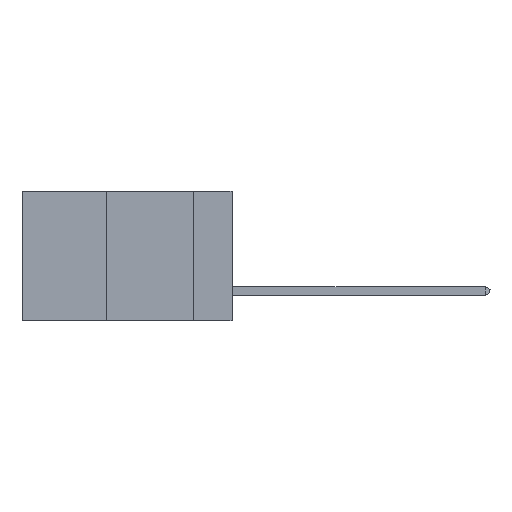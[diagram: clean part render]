
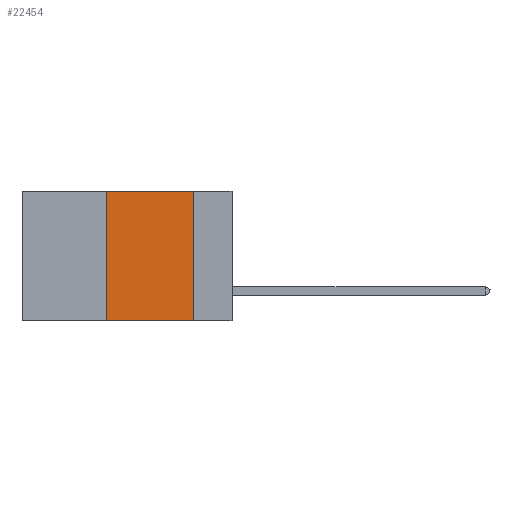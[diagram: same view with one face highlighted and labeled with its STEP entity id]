
A CAD part, left-side view. The second image highlights one B-rep face of the part: STEP entity #22454.
In plain terms, the highlighted planar face has unit normal (-1, 0, 0).
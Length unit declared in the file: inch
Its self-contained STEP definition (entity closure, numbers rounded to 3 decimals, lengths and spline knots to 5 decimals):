
#718 = AXIS2_PLACEMENT_3D ( 'NONE', #11812, #4247, #4159 ) ;
#1713 = VECTOR ( 'NONE', #14439, 39.37008 ) ;
#2725 = VERTEX_POINT ( 'NONE', #11721 ) ;
#4064 = DIRECTION ( 'NONE',  ( 0., 0., -1. ) ) ;
#4159 = DIRECTION ( 'NONE',  ( 0., 0., -1. ) ) ;
#4247 = DIRECTION ( 'NONE',  ( 1., 0., 0. ) ) ;
#4410 = PLANE ( 'NONE',  #718 ) ;
#4430 = VERTEX_POINT ( 'NONE', #20832 ) ;
#6059 = CARTESIAN_POINT ( 'NONE',  ( 0., 0.11, 0. ) ) ;
#7761 = ORIENTED_EDGE ( 'NONE', *, *, #22432, .F. ) ;
#8050 = EDGE_CURVE ( 'NONE', #13693, #23708, #11525, .T. ) ;
#8743 = LINE ( 'NONE', #18238, #1713 ) ;
#9168 = CARTESIAN_POINT ( 'NONE',  ( 0., 0.36, -0.37 ) ) ;
#9660 = ORIENTED_EDGE ( 'NONE', *, *, #18274, .F. ) ;
#10077 = DIRECTION ( 'NONE',  ( 0., 0., 1. ) ) ;
#11281 = FACE_OUTER_BOUND ( 'NONE', #19288, .T. ) ;
#11525 = LINE ( 'NONE', #17593, #18922 ) ;
#11721 = CARTESIAN_POINT ( 'NONE',  ( 0., 0.36, 0. ) ) ;
#11812 = CARTESIAN_POINT ( 'NONE',  ( 0., 0.6, 0. ) ) ;
#12794 = LINE ( 'NONE', #15980, #19209 ) ;
#12818 = VECTOR ( 'NONE', #4064, 39.37008 ) ;
#13693 = VERTEX_POINT ( 'NONE', #9168 ) ;
#14439 = DIRECTION ( 'NONE',  ( 0., -1., 0. ) ) ;
#15980 = CARTESIAN_POINT ( 'NONE',  ( 0., 0.36, 0. ) ) ;
#16267 = ORIENTED_EDGE ( 'NONE', *, *, #8050, .T. ) ;
#17593 = CARTESIAN_POINT ( 'NONE',  ( 0., 0.6, -0.37 ) ) ;
#18238 = CARTESIAN_POINT ( 'NONE',  ( 0., 0.6, 0. ) ) ;
#18274 = EDGE_CURVE ( 'NONE', #2725, #4430, #8743, .T. ) ;
#18922 = VECTOR ( 'NONE', #19159, 39.37008 ) ;
#19159 = DIRECTION ( 'NONE',  ( 0., -1., 0. ) ) ;
#19209 = VECTOR ( 'NONE', #10077, 39.37008 ) ;
#19288 = EDGE_LOOP ( 'NONE', ( #7761, #9660, #19575, #16267 ) ) ;
#19575 = ORIENTED_EDGE ( 'NONE', *, *, #21214, .F. ) ;
#20358 = CARTESIAN_POINT ( 'NONE',  ( 0., 0.11, -0.37 ) ) ;
#20832 = CARTESIAN_POINT ( 'NONE',  ( 0., 0.11, 0. ) ) ;
#21214 = EDGE_CURVE ( 'NONE', #13693, #2725, #12794, .T. ) ;
#22432 = EDGE_CURVE ( 'NONE', #4430, #23708, #23851, .T. ) ;
#22454 = ADVANCED_FACE ( 'NONE', ( #11281 ), #4410, .F. ) ;
#23708 = VERTEX_POINT ( 'NONE', #20358 ) ;
#23851 = LINE ( 'NONE', #6059, #12818 ) ;
